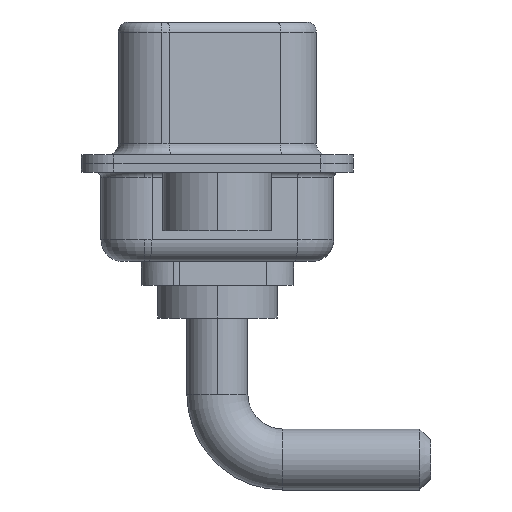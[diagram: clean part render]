
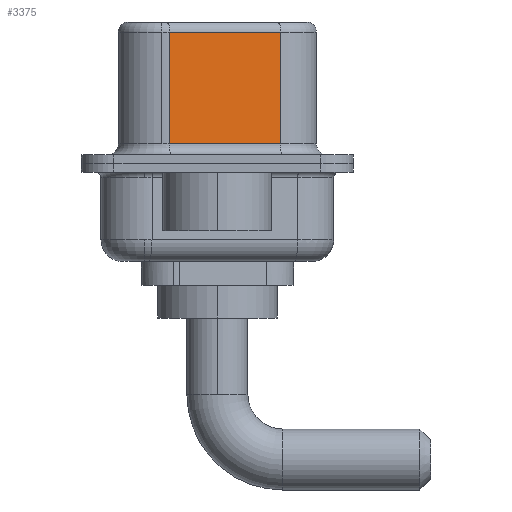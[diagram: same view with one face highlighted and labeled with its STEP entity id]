
A CAD part, left-side view. The second image highlights one B-rep face of the part: STEP entity #3375.
In plain terms, the highlighted planar face has unit normal (-0.985, -0.174, 0).
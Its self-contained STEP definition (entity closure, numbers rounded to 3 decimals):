
#696 = EDGE_CURVE ( 'NONE', #7531, #1911, #10468, .T. ) ;
#1301 = ORIENTED_EDGE ( 'NONE', *, *, #12679, .T. ) ;
#1546 = CARTESIAN_POINT ( 'NONE',  ( 3.68, 2.203, 0.9 ) ) ;
#1911 = VERTEX_POINT ( 'NONE', #14432 ) ;
#2433 = EDGE_CURVE ( 'NONE', #7531, #11779, #12871, .T. ) ;
#2690 = FACE_OUTER_BOUND ( 'NONE', #12776, .T. ) ;
#2976 = VERTEX_POINT ( 'NONE', #1546 ) ;
#3375 = ADVANCED_FACE ( 'NONE', ( #2690 ), #8245, .F. ) ;
#3587 = ORIENTED_EDGE ( 'NONE', *, *, #2433, .T. ) ;
#3954 = CARTESIAN_POINT ( 'NONE',  ( 4.58, -2.897, 6.02 ) ) ;
#4071 = CARTESIAN_POINT ( 'NONE',  ( 4.58, -2.897, 0.9 ) ) ;
#4287 = EDGE_CURVE ( 'NONE', #11779, #2976, #13957, .T. ) ;
#4316 = VECTOR ( 'NONE', #13531, 1000. ) ;
#4368 = VECTOR ( 'NONE', #7181, 1000. ) ;
#5965 = ORIENTED_EDGE ( 'NONE', *, *, #4287, .T. ) ;
#5992 = CARTESIAN_POINT ( 'NONE',  ( 4.58, -2.897, 6.52 ) ) ;
#6405 = AXIS2_PLACEMENT_3D ( 'NONE', #9338, #8101, #13566 ) ;
#6498 = VECTOR ( 'NONE', #7108, 1000. ) ;
#7108 = DIRECTION ( 'NONE',  ( 0., 0., -1. ) ) ;
#7181 = DIRECTION ( 'NONE',  ( -0.174, 0.985, 0. ) ) ;
#7531 = VERTEX_POINT ( 'NONE', #12559 ) ;
#8101 = DIRECTION ( 'NONE',  ( 0.985, 0.174, 0. ) ) ;
#8245 = PLANE ( 'NONE',  #6405 ) ;
#8879 = CARTESIAN_POINT ( 'NONE',  ( 3.68, 2.203, 6.02 ) ) ;
#9338 = CARTESIAN_POINT ( 'NONE',  ( 4.58, -2.897, 6.52 ) ) ;
#10468 = LINE ( 'NONE', #5992, #6498 ) ;
#10583 = DIRECTION ( 'NONE',  ( 0.174, -0.985, 0. ) ) ;
#11424 = CARTESIAN_POINT ( 'NONE',  ( 3.68, 2.203, 6.52 ) ) ;
#11779 = VERTEX_POINT ( 'NONE', #8879 ) ;
#12559 = CARTESIAN_POINT ( 'NONE',  ( 4.58, -2.897, 6.02 ) ) ;
#12679 = EDGE_CURVE ( 'NONE', #2976, #1911, #14089, .T. ) ;
#12776 = EDGE_LOOP ( 'NONE', ( #13979, #3587, #5965, #1301 ) ) ;
#12871 = LINE ( 'NONE', #3954, #4368 ) ;
#13531 = DIRECTION ( 'NONE',  ( 0., 0., -1. ) ) ;
#13566 = DIRECTION ( 'NONE',  ( -0.174, 0.985, 0. ) ) ;
#13794 = VECTOR ( 'NONE', #10583, 1000. ) ;
#13957 = LINE ( 'NONE', #11424, #4316 ) ;
#13979 = ORIENTED_EDGE ( 'NONE', *, *, #696, .F. ) ;
#14089 = LINE ( 'NONE', #4071, #13794 ) ;
#14432 = CARTESIAN_POINT ( 'NONE',  ( 4.58, -2.897, 0.9 ) ) ;
